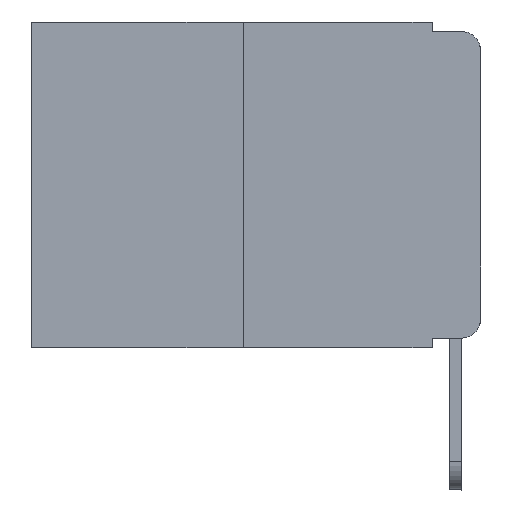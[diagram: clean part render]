
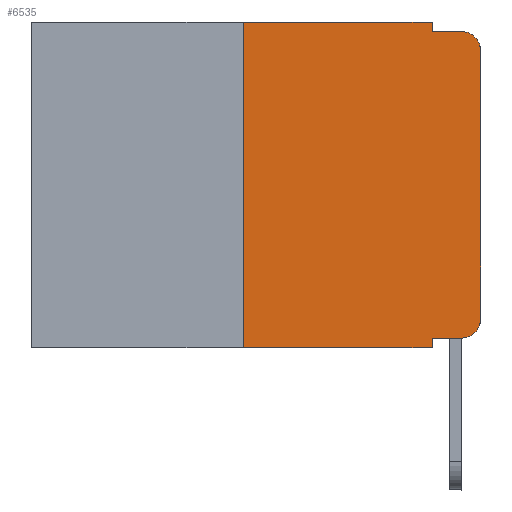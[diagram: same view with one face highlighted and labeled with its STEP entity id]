
A CAD part, left-side view. The second image highlights one B-rep face of the part: STEP entity #6535.
In plain terms, the highlighted planar face has unit normal (-1, 0, 0).
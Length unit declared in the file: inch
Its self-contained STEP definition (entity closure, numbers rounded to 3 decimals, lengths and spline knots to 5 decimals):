
#216 = CARTESIAN_POINT ( 'NONE',  ( 0., 0., -0.03 ) ) ;
#229 = VERTEX_POINT ( 'NONE', #17890 ) ;
#341 = VERTEX_POINT ( 'NONE', #216 ) ;
#488 = PLANE ( 'NONE',  #504 ) ;
#504 = AXIS2_PLACEMENT_3D ( 'NONE', #13259, #9735, #16177 ) ;
#518 = EDGE_CURVE ( 'NONE', #7298, #229, #18599, .T. ) ;
#816 = VECTOR ( 'NONE', #15154, 39.37008 ) ;
#838 = CARTESIAN_POINT ( 'NONE',  ( 0., 0.051, -0.333 ) ) ;
#1173 = LINE ( 'NONE', #9372, #19786 ) ;
#1546 = ORIENTED_EDGE ( 'NONE', *, *, #11811, .T. ) ;
#1992 = VERTEX_POINT ( 'NONE', #9930 ) ;
#2695 = LINE ( 'NONE', #4466, #18170 ) ;
#2802 = DIRECTION ( 'NONE',  ( 0., -1., 0. ) ) ;
#2841 = DIRECTION ( 'NONE',  ( 0., 0., -1. ) ) ;
#2939 = DIRECTION ( 'NONE',  ( 0., 0., -1. ) ) ;
#3119 = DIRECTION ( 'NONE',  ( 0., 0., 1. ) ) ;
#3321 = CARTESIAN_POINT ( 'NONE',  ( 0., 0.473, 0. ) ) ;
#3511 = ORIENTED_EDGE ( 'NONE', *, *, #12734, .F. ) ;
#4357 = CARTESIAN_POINT ( 'NONE',  ( 0., 0.02, -0.03 ) ) ;
#4432 = VERTEX_POINT ( 'NONE', #11368 ) ;
#4466 = CARTESIAN_POINT ( 'NONE',  ( 0., 0.473, -0.343 ) ) ;
#4599 = CARTESIAN_POINT ( 'NONE',  ( 0., 0.051, -0.343 ) ) ;
#4629 = CARTESIAN_POINT ( 'NONE',  ( 0., 0.051, -0.01 ) ) ;
#4697 = CARTESIAN_POINT ( 'NONE',  ( 0., 0.25, -0.343 ) ) ;
#4952 = VERTEX_POINT ( 'NONE', #18108 ) ;
#5012 = ORIENTED_EDGE ( 'NONE', *, *, #20019, .T. ) ;
#5287 = CARTESIAN_POINT ( 'NONE',  ( 0., 0.051, 0. ) ) ;
#5503 = VECTOR ( 'NONE', #17188, 39.37008 ) ;
#5510 = DIRECTION ( 'NONE',  ( 0., 0., 1. ) ) ;
#5720 = LINE ( 'NONE', #838, #816 ) ;
#5765 = EDGE_CURVE ( 'NONE', #341, #4432, #9752, .T. ) ;
#6098 = ORIENTED_EDGE ( 'NONE', *, *, #14116, .F. ) ;
#6535 = ADVANCED_FACE ( 'NONE', ( #6955 ), #488, .F. ) ;
#6955 = FACE_OUTER_BOUND ( 'NONE', #10679, .T. ) ;
#6973 = CARTESIAN_POINT ( 'NONE',  ( 0., 0.02, -0.313 ) ) ;
#7165 = DIRECTION ( 'NONE',  ( 0., 0., -1. ) ) ;
#7292 = EDGE_CURVE ( 'NONE', #12444, #1992, #1173, .T. ) ;
#7298 = VERTEX_POINT ( 'NONE', #4697 ) ;
#7674 = LINE ( 'NONE', #3321, #10028 ) ;
#7996 = ORIENTED_EDGE ( 'NONE', *, *, #518, .F. ) ;
#8088 = AXIS2_PLACEMENT_3D ( 'NONE', #4357, #16721, #13807 ) ;
#9372 = CARTESIAN_POINT ( 'NONE',  ( 0., 0.051, 0. ) ) ;
#9735 = DIRECTION ( 'NONE',  ( 1., 0., 0. ) ) ;
#9752 = CIRCLE ( 'NONE', #8088, 0.02 ) ;
#9930 = CARTESIAN_POINT ( 'NONE',  ( 0., 0.051, -0.01 ) ) ;
#10028 = VECTOR ( 'NONE', #19109, 39.37008 ) ;
#10527 = EDGE_CURVE ( 'NONE', #229, #12444, #7674, .T. ) ;
#10679 = EDGE_LOOP ( 'NONE', ( #16963, #10811, #3511, #16003, #18803, #7996, #14986, #6098, #1546, #5012 ) ) ;
#10811 = ORIENTED_EDGE ( 'NONE', *, *, #5765, .T. ) ;
#11106 = CARTESIAN_POINT ( 'NONE',  ( 0., 0.25, 0. ) ) ;
#11368 = CARTESIAN_POINT ( 'NONE',  ( 0., 0.02, -0.01 ) ) ;
#11509 = VERTEX_POINT ( 'NONE', #4599 ) ;
#11811 = EDGE_CURVE ( 'NONE', #12363, #13111, #5720, .T. ) ;
#12363 = VERTEX_POINT ( 'NONE', #18981 ) ;
#12444 = VERTEX_POINT ( 'NONE', #5287 ) ;
#12734 = EDGE_CURVE ( 'NONE', #1992, #4432, #15518, .T. ) ;
#13111 = VERTEX_POINT ( 'NONE', #15569 ) ;
#13259 = CARTESIAN_POINT ( 'NONE',  ( 0., 0.473, 0. ) ) ;
#13381 = LINE ( 'NONE', #19743, #15779 ) ;
#13382 = EDGE_CURVE ( 'NONE', #4952, #341, #13381, .T. ) ;
#13544 = VECTOR ( 'NONE', #3119, 39.37008 ) ;
#13807 = DIRECTION ( 'NONE',  ( 0., 0., -1. ) ) ;
#14116 = EDGE_CURVE ( 'NONE', #12363, #11509, #19021, .T. ) ;
#14986 = ORIENTED_EDGE ( 'NONE', *, *, #17392, .T. ) ;
#15154 = DIRECTION ( 'NONE',  ( 0., -1., 0. ) ) ;
#15518 = LINE ( 'NONE', #4629, #5503 ) ;
#15569 = CARTESIAN_POINT ( 'NONE',  ( 0., 0.02, -0.333 ) ) ;
#15779 = VECTOR ( 'NONE', #5510, 39.37008 ) ;
#16003 = ORIENTED_EDGE ( 'NONE', *, *, #7292, .F. ) ;
#16177 = DIRECTION ( 'NONE',  ( 0., 0., -1. ) ) ;
#16721 = DIRECTION ( 'NONE',  ( -1., 0., 0. ) ) ;
#16963 = ORIENTED_EDGE ( 'NONE', *, *, #13382, .T. ) ;
#17178 = CIRCLE ( 'NONE', #19855, 0.02 ) ;
#17188 = DIRECTION ( 'NONE',  ( 0., -1., 0. ) ) ;
#17392 = EDGE_CURVE ( 'NONE', #7298, #11509, #2695, .T. ) ;
#17890 = CARTESIAN_POINT ( 'NONE',  ( 0., 0.25, 0. ) ) ;
#17969 = DIRECTION ( 'NONE',  ( -1., 0., 0. ) ) ;
#18108 = CARTESIAN_POINT ( 'NONE',  ( 0., 0., -0.313 ) ) ;
#18170 = VECTOR ( 'NONE', #2802, 39.37008 ) ;
#18599 = LINE ( 'NONE', #11106, #13544 ) ;
#18722 = CARTESIAN_POINT ( 'NONE',  ( 0., 0.051, 0. ) ) ;
#18765 = VECTOR ( 'NONE', #2939, 39.37008 ) ;
#18803 = ORIENTED_EDGE ( 'NONE', *, *, #10527, .F. ) ;
#18981 = CARTESIAN_POINT ( 'NONE',  ( 0., 0.051, -0.333 ) ) ;
#19021 = LINE ( 'NONE', #18722, #18765 ) ;
#19109 = DIRECTION ( 'NONE',  ( 0., -1., 0. ) ) ;
#19743 = CARTESIAN_POINT ( 'NONE',  ( 0., 0., 0. ) ) ;
#19786 = VECTOR ( 'NONE', #2841, 39.37008 ) ;
#19855 = AXIS2_PLACEMENT_3D ( 'NONE', #6973, #17969, #7165 ) ;
#20019 = EDGE_CURVE ( 'NONE', #13111, #4952, #17178, .T. ) ;
